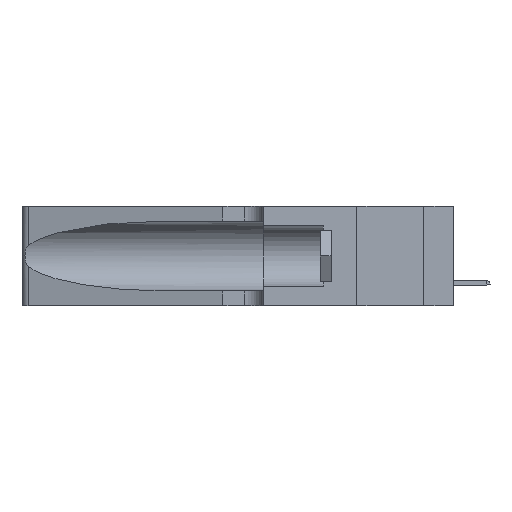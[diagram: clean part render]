
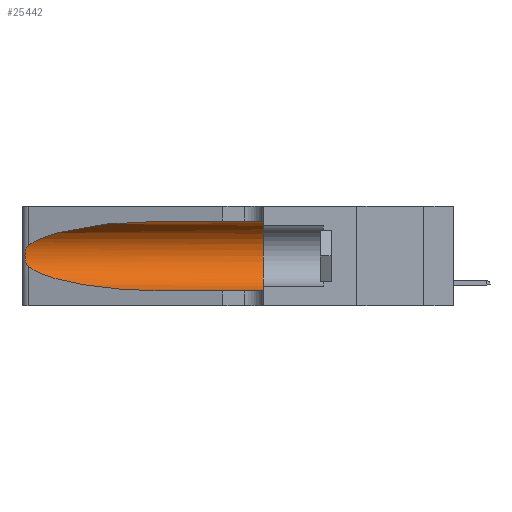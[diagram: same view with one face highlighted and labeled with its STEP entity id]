
A CAD part, left-side view. The second image highlights one B-rep face of the part: STEP entity #25442.
In plain terms, the highlighted cylindrical face has radius 3.308 mm (diameter 6.617 mm), a partial arc.
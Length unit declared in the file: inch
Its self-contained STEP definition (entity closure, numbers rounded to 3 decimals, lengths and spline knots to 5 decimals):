
#546 = CARTESIAN_POINT ( 'NONE',  ( 0.2373, 1.15595, 0.08982 ) ) ;
#749 = VERTEX_POINT ( 'NONE', #12301 ) ;
#810 = DIRECTION ( 'NONE',  ( 0., -1., 0. ) ) ;
#1398 = EDGE_CURVE ( 'NONE', #35990, #13759, #24307, .T. ) ;
#2129 = EDGE_CURVE ( 'NONE', #13759, #37269, #34414, .T. ) ;
#3034 = CARTESIAN_POINT ( 'NONE',  ( 0.25639, 1.23186, 0.15144 ) ) ;
#3244 = CARTESIAN_POINT ( 'NONE',  ( 0.25789, 1.23486, 0.15765 ) ) ;
#4303 = CARTESIAN_POINT ( 'NONE',  ( 0.2373, 1.15595, 0.28018 ) ) ;
#5687 = CARTESIAN_POINT ( 'NONE',  ( 0.1305, 0.35, 0.31525 ) ) ;
#6742 = CARTESIAN_POINT ( 'NONE',  ( 0.1305, 1.61858, 0.31525 ) ) ;
#6879 = CARTESIAN_POINT ( 'NONE',  ( 0.25487, 1.22718, 0.22369 ) ) ;
#7129 = CARTESIAN_POINT ( 'NONE',  ( 0.1305, 1.61858, 0.185 ) ) ;
#7615 = CARTESIAN_POINT ( 'NONE',  ( 0.25555, 1.22994, 0.2215 ) ) ;
#9645 = CARTESIAN_POINT ( 'NONE',  ( 0.1305, 0.72297, 0.31525 ) ) ;
#11142 = CARTESIAN_POINT ( 'NONE',  ( 0.26075, 1.23896, 0.178 ) ) ;
#11151 = ORIENTED_EDGE ( 'NONE', *, *, #34580, .F. ) ;
#11805 = DIRECTION ( 'NONE',  ( 0., 0., 1. ) ) ;
#12301 = CARTESIAN_POINT ( 'NONE',  ( 0.1305, 0.35, 0.05475 ) ) ;
#12576 = CARTESIAN_POINT ( 'NONE',  ( 0.18966, 0.96281, 0.05475 ) ) ;
#13759 = VERTEX_POINT ( 'NONE', #36453 ) ;
#14219 = EDGE_CURVE ( 'NONE', #37269, #28487, #28101, .T. ) ;
#14470 = CARTESIAN_POINT ( 'NONE',  ( 0.25487, 1.22718, 0.14631 ) ) ;
#14805 = EDGE_CURVE ( 'NONE', #28487, #749, #19340, .T. ) ;
#14876 = ORIENTED_EDGE ( 'NONE', *, *, #36185, .F. ) ;
#16116 = CARTESIAN_POINT ( 'NONE',  ( 0.1305, 0.72297, 0.05475 ) ) ;
#16445 = CARTESIAN_POINT ( 'NONE',  ( 0.26017, 1.23833, 0.17102 ) ) ;
#17684 = VERTEX_POINT ( 'NONE', #5687 ) ;
#18774 = CIRCLE ( 'NONE', #23808, 0.13025 ) ;
#19115 = DIRECTION ( 'NONE',  ( 0., -1., 0. ) ) ;
#19340 = LINE ( 'NONE', #25858, #27178 ) ;
#19607 = CARTESIAN_POINT ( 'NONE',  ( 0.25787, 1.23484, 0.2124 ) ) ;
#19702 = FACE_OUTER_BOUND ( 'NONE', #36631, .T. ) ;
#20190 = CARTESIAN_POINT ( 'NONE',  ( 0.25639, 1.23184, 0.21858 ) ) ;
#20858 = CARTESIAN_POINT ( 'NONE',  ( 0.1305, 0.72297, 0.05475 ) ) ;
#21459 = DIRECTION ( 'NONE',  ( 0., 1., 0. ) ) ;
#22779 = ORIENTED_EDGE ( 'NONE', *, *, #14805, .T. ) ;
#23679 = CARTESIAN_POINT ( 'NONE',  ( 0.25487, 1.22718, 0.14631 ) ) ;
#23808 = AXIS2_PLACEMENT_3D ( 'NONE', #36412, #21459, #11805 ) ;
#24307 =( BOUNDED_CURVE ( )  B_SPLINE_CURVE ( 3, ( #9645, #31475, #4303, #6879 ),
 .UNSPECIFIED., .F., .F. ) 
 B_SPLINE_CURVE_WITH_KNOTS ( ( 4, 4 ),
 ( 1.5708, 2.84003 ),
 .UNSPECIFIED. ) 
 CURVE ( )  GEOMETRIC_REPRESENTATION_ITEM ( )  RATIONAL_B_SPLINE_CURVE ( ( 1., 0.87, 0.87, 1. ) ) 
 REPRESENTATION_ITEM ( '' )  );
#25442 = ADVANCED_FACE ( 'NONE', ( #19702 ), #34101, .F. ) ;
#25858 = CARTESIAN_POINT ( 'NONE',  ( 0.1305, 1.61858, 0.05475 ) ) ;
#26110 = CARTESIAN_POINT ( 'NONE',  ( 0.25487, 1.22718, 0.22369 ) ) ;
#26442 = CARTESIAN_POINT ( 'NONE',  ( 0.1305, 0.72297, 0.31525 ) ) ;
#27178 = VECTOR ( 'NONE', #31762, 39.37008 ) ;
#27697 = VECTOR ( 'NONE', #810, 39.37008 ) ;
#28101 =( BOUNDED_CURVE ( )  B_SPLINE_CURVE ( 3, ( #30105, #546, #12576, #20858 ),
 .UNSPECIFIED., .F., .F. ) 
 B_SPLINE_CURVE_WITH_KNOTS ( ( 4, 4 ),
 ( 3.44316, 4.71239 ),
 .UNSPECIFIED. ) 
 CURVE ( )  GEOMETRIC_REPRESENTATION_ITEM ( )  RATIONAL_B_SPLINE_CURVE ( ( 1., 0.87, 0.87, 1. ) ) 
 REPRESENTATION_ITEM ( '' )  );
#28487 = VERTEX_POINT ( 'NONE', #16116 ) ;
#29163 = AXIS2_PLACEMENT_3D ( 'NONE', #7129, #19115, #37623 ) ;
#29214 = ORIENTED_EDGE ( 'NONE', *, *, #14219, .T. ) ;
#29251 = CARTESIAN_POINT ( 'NONE',  ( 0.25856, 1.23593, 0.16098 ) ) ;
#30105 = CARTESIAN_POINT ( 'NONE',  ( 0.25487, 1.22718, 0.14631 ) ) ;
#30864 = ORIENTED_EDGE ( 'NONE', *, *, #1398, .T. ) ;
#31421 = CARTESIAN_POINT ( 'NONE',  ( 0.25854, 1.2359, 0.20912 ) ) ;
#31475 = CARTESIAN_POINT ( 'NONE',  ( 0.18966, 0.96281, 0.31525 ) ) ;
#31762 = DIRECTION ( 'NONE',  ( 0., -1., 0. ) ) ;
#32217 = CARTESIAN_POINT ( 'NONE',  ( 0.26075, 1.23896, 0.19203 ) ) ;
#33711 = LINE ( 'NONE', #6742, #27697 ) ;
#34101 = CYLINDRICAL_SURFACE ( 'NONE', #29163, 0.13025 ) ;
#34414 = B_SPLINE_CURVE_WITH_KNOTS ( 'NONE', 3,
 ( #26110, #7615, #20190, #19607, #31421, #38108, #32217, #11142, #16445, #29251, #3244, #3034, #38870, #14470 ),
 .UNSPECIFIED., .F., .F.,
 ( 4, 2, 2, 2, 2, 2, 4 ),
 ( 0., 0.00027, 0.00053, 0.00107, 0.0016, 0.00187, 0.00214 ),
 .UNSPECIFIED. ) ;
#34580 = EDGE_CURVE ( 'NONE', #17684, #749, #18774, .T. ) ;
#35990 = VERTEX_POINT ( 'NONE', #26442 ) ;
#36108 = ORIENTED_EDGE ( 'NONE', *, *, #2129, .T. ) ;
#36185 = EDGE_CURVE ( 'NONE', #35990, #17684, #33711, .T. ) ;
#36412 = CARTESIAN_POINT ( 'NONE',  ( 0.1305, 0.35, 0.185 ) ) ;
#36453 = CARTESIAN_POINT ( 'NONE',  ( 0.25487, 1.22718, 0.22369 ) ) ;
#36631 = EDGE_LOOP ( 'NONE', ( #30864, #36108, #29214, #22779, #11151, #14876 ) ) ;
#37269 = VERTEX_POINT ( 'NONE', #23679 ) ;
#37623 = DIRECTION ( 'NONE',  ( 0., 0., -1. ) ) ;
#38108 = CARTESIAN_POINT ( 'NONE',  ( 0.26018, 1.23835, 0.19895 ) ) ;
#38870 = CARTESIAN_POINT ( 'NONE',  ( 0.25555, 1.22993, 0.14849 ) ) ;
